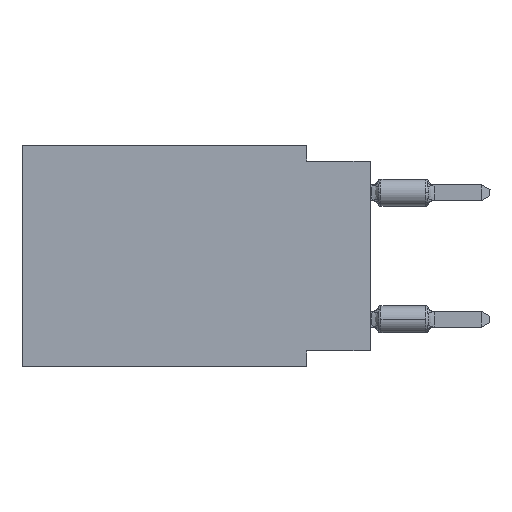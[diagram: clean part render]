
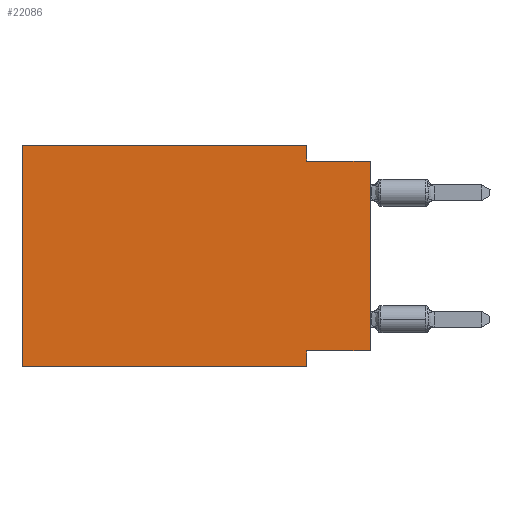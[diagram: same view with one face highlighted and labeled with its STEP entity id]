
A CAD part, left-side view. The second image highlights one B-rep face of the part: STEP entity #22086.
In plain terms, the highlighted planar face has unit normal (-1, 0, 0).
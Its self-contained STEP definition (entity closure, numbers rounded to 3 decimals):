
#793 = EDGE_LOOP ( 'NONE', ( #22105, #41229, #42647, #19422, #46346, #32568, #28911, #4799 ) ) ;
#1751 = VECTOR ( 'NONE', #40401, 1000. ) ;
#3937 = CARTESIAN_POINT ( 'NONE',  ( 0., 0., -0.635 ) ) ;
#4799 = ORIENTED_EDGE ( 'NONE', *, *, #37052, .F. ) ;
#4877 = CARTESIAN_POINT ( 'NONE',  ( 0., 13.97, 0. ) ) ;
#5650 = DIRECTION ( 'NONE',  ( 0., 0., 1. ) ) ;
#7336 = VECTOR ( 'NONE', #21236, 1000. ) ;
#7545 = AXIS2_PLACEMENT_3D ( 'NONE', #26069, #17492, #13712 ) ;
#9259 = VERTEX_POINT ( 'NONE', #38761 ) ;
#9555 = DIRECTION ( 'NONE',  ( 0., -1., 0. ) ) ;
#9589 = LINE ( 'NONE', #24983, #1751 ) ;
#10113 = LINE ( 'NONE', #18417, #46925 ) ;
#10198 = LINE ( 'NONE', #28864, #42334 ) ;
#13467 = PLANE ( 'NONE',  #7545 ) ;
#13712 = DIRECTION ( 'NONE',  ( 0., 0., -1. ) ) ;
#15211 = VERTEX_POINT ( 'NONE', #3937 ) ;
#15951 = DIRECTION ( 'NONE',  ( 0., 0., 1. ) ) ;
#16274 = LINE ( 'NONE', #20311, #42441 ) ;
#17181 = CARTESIAN_POINT ( 'NONE',  ( 0., 2.54, -0.635 ) ) ;
#17492 = DIRECTION ( 'NONE',  ( 1., 0., 0. ) ) ;
#18417 = CARTESIAN_POINT ( 'NONE',  ( 0., 2.54, 0. ) ) ;
#18657 = VECTOR ( 'NONE', #15951, 1000. ) ;
#19422 = ORIENTED_EDGE ( 'NONE', *, *, #35179, .F. ) ;
#20311 = CARTESIAN_POINT ( 'NONE',  ( 0., 0., -8.255 ) ) ;
#21236 = DIRECTION ( 'NONE',  ( 0., -1., 0. ) ) ;
#21550 = CARTESIAN_POINT ( 'NONE',  ( 0., 2.54, -8.255 ) ) ;
#21667 = CARTESIAN_POINT ( 'NONE',  ( 0., 0., -0.635 ) ) ;
#22086 = ADVANCED_FACE ( 'NONE', ( #41228 ), #13467, .F. ) ;
#22105 = ORIENTED_EDGE ( 'NONE', *, *, #28052, .T. ) ;
#22395 = LINE ( 'NONE', #37801, #24560 ) ;
#24560 = VECTOR ( 'NONE', #29480, 1000. ) ;
#24983 = CARTESIAN_POINT ( 'NONE',  ( 0., 2.54, -8.89 ) ) ;
#25268 = LINE ( 'NONE', #40670, #7336 ) ;
#26069 = CARTESIAN_POINT ( 'NONE',  ( 0., 13.97, 0. ) ) ;
#26326 = CARTESIAN_POINT ( 'NONE',  ( 0., 2.54, 0. ) ) ;
#26849 = VERTEX_POINT ( 'NONE', #26326 ) ;
#27900 = VECTOR ( 'NONE', #9555, 1000. ) ;
#28052 = EDGE_CURVE ( 'NONE', #9259, #15211, #33730, .T. ) ;
#28864 = CARTESIAN_POINT ( 'NONE',  ( 0., 13.97, 0. ) ) ;
#28876 = CARTESIAN_POINT ( 'NONE',  ( 0., 2.54, -8.89 ) ) ;
#28911 = ORIENTED_EDGE ( 'NONE', *, *, #41611, .F. ) ;
#29480 = DIRECTION ( 'NONE',  ( 0., -1., 0. ) ) ;
#29676 = VERTEX_POINT ( 'NONE', #28876 ) ;
#32025 = VERTEX_POINT ( 'NONE', #17181 ) ;
#32131 = EDGE_CURVE ( 'NONE', #26849, #32025, #10113, .T. ) ;
#32547 = LINE ( 'NONE', #21667, #27900 ) ;
#32568 = ORIENTED_EDGE ( 'NONE', *, *, #49628, .T. ) ;
#33730 = LINE ( 'NONE', #49138, #18657 ) ;
#35179 = EDGE_CURVE ( 'NONE', #47832, #26849, #22395, .T. ) ;
#35935 = EDGE_CURVE ( 'NONE', #48273, #47832, #10198, .T. ) ;
#35942 = VERTEX_POINT ( 'NONE', #21550 ) ;
#36855 = EDGE_CURVE ( 'NONE', #32025, #15211, #32547, .T. ) ;
#37052 = EDGE_CURVE ( 'NONE', #9259, #35942, #16274, .T. ) ;
#37801 = CARTESIAN_POINT ( 'NONE',  ( 0., 13.97, 0. ) ) ;
#38761 = CARTESIAN_POINT ( 'NONE',  ( 0., 0., -8.255 ) ) ;
#40401 = DIRECTION ( 'NONE',  ( 0., 0., -1. ) ) ;
#40670 = CARTESIAN_POINT ( 'NONE',  ( 0., 13.97, -8.89 ) ) ;
#41228 = FACE_OUTER_BOUND ( 'NONE', #793, .T. ) ;
#41229 = ORIENTED_EDGE ( 'NONE', *, *, #36855, .F. ) ;
#41611 = EDGE_CURVE ( 'NONE', #35942, #29676, #9589, .T. ) ;
#42334 = VECTOR ( 'NONE', #5650, 1000. ) ;
#42441 = VECTOR ( 'NONE', #43527, 1000. ) ;
#42647 = ORIENTED_EDGE ( 'NONE', *, *, #32131, .F. ) ;
#43527 = DIRECTION ( 'NONE',  ( 0., 1., 0. ) ) ;
#44942 = DIRECTION ( 'NONE',  ( 0., 0., -1. ) ) ;
#46346 = ORIENTED_EDGE ( 'NONE', *, *, #35935, .F. ) ;
#46925 = VECTOR ( 'NONE', #44942, 1000. ) ;
#47475 = CARTESIAN_POINT ( 'NONE',  ( 0., 13.97, -8.89 ) ) ;
#47832 = VERTEX_POINT ( 'NONE', #4877 ) ;
#48273 = VERTEX_POINT ( 'NONE', #47475 ) ;
#49138 = CARTESIAN_POINT ( 'NONE',  ( 0., 0., 0. ) ) ;
#49628 = EDGE_CURVE ( 'NONE', #48273, #29676, #25268, .T. ) ;
